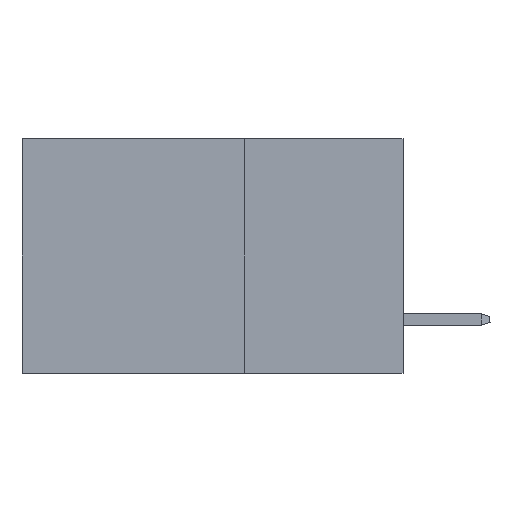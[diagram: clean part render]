
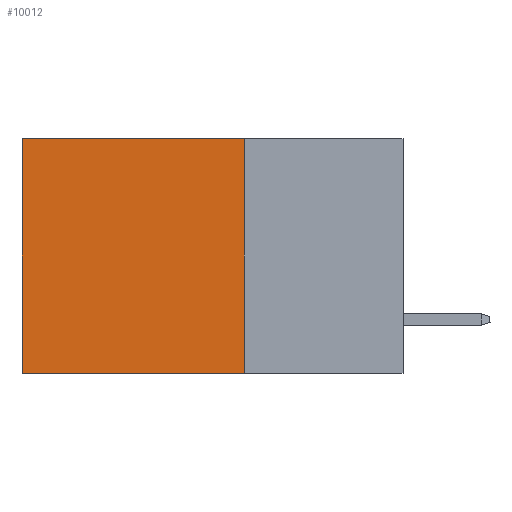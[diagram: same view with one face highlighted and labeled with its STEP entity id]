
A CAD part, left-side view. The second image highlights one B-rep face of the part: STEP entity #10012.
In plain terms, the highlighted planar face has unit normal (-1, 0, 0).
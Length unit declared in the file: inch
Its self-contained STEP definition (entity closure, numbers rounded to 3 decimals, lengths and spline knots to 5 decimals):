
#1174 = DIRECTION ( 'NONE',  ( 0., 1., 0. ) ) ;
#1626 = VERTEX_POINT ( 'NONE', #35680 ) ;
#2067 = LINE ( 'NONE', #16217, #13193 ) ;
#4987 = VECTOR ( 'NONE', #1174, 39.37008 ) ;
#7711 = CARTESIAN_POINT ( 'NONE',  ( 0.2875, 0.25, 0. ) ) ;
#7840 = EDGE_CURVE ( 'NONE', #28309, #1626, #2067, .T. ) ;
#8248 = CARTESIAN_POINT ( 'NONE',  ( 0.2875, 0.25, 0. ) ) ;
#9407 = DIRECTION ( 'NONE',  ( 0., 0., -1. ) ) ;
#9444 = CARTESIAN_POINT ( 'NONE',  ( 0.2875, 0.6, -0.37 ) ) ;
#10012 = ADVANCED_FACE ( 'NONE', ( #19059 ), #16410, .F. ) ;
#12593 = LINE ( 'NONE', #29632, #17656 ) ;
#12969 = DIRECTION ( 'NONE',  ( 0., 1., 0. ) ) ;
#13193 = VECTOR ( 'NONE', #36003, 39.37008 ) ;
#13343 = CARTESIAN_POINT ( 'NONE',  ( 0.2875, 0.25, 0. ) ) ;
#14659 = EDGE_CURVE ( 'NONE', #28309, #22781, #18462, .T. ) ;
#15613 = CARTESIAN_POINT ( 'NONE',  ( 0.2875, 0.6, 0. ) ) ;
#15822 = EDGE_CURVE ( 'NONE', #22781, #23527, #12593, .T. ) ;
#16217 = CARTESIAN_POINT ( 'NONE',  ( 0.2875, 0.25, 0. ) ) ;
#16410 = PLANE ( 'NONE',  #28434 ) ;
#17656 = VECTOR ( 'NONE', #9407, 39.37008 ) ;
#18462 = LINE ( 'NONE', #13343, #32437 ) ;
#19059 = FACE_OUTER_BOUND ( 'NONE', #37117, .T. ) ;
#19250 = DIRECTION ( 'NONE',  ( 0., 0., -1. ) ) ;
#22781 = VERTEX_POINT ( 'NONE', #15613 ) ;
#23527 = VERTEX_POINT ( 'NONE', #9444 ) ;
#27048 = CARTESIAN_POINT ( 'NONE',  ( 0.2875, 0.25, -0.37 ) ) ;
#28309 = VERTEX_POINT ( 'NONE', #8248 ) ;
#28434 = AXIS2_PLACEMENT_3D ( 'NONE', #7711, #36937, #19250 ) ;
#29013 = ORIENTED_EDGE ( 'NONE', *, *, #7840, .F. ) ;
#29632 = CARTESIAN_POINT ( 'NONE',  ( 0.2875, 0.6, 0. ) ) ;
#32437 = VECTOR ( 'NONE', #12969, 39.37008 ) ;
#32863 = LINE ( 'NONE', #27048, #4987 ) ;
#33533 = ORIENTED_EDGE ( 'NONE', *, *, #36767, .F. ) ;
#33641 = ORIENTED_EDGE ( 'NONE', *, *, #15822, .T. ) ;
#35680 = CARTESIAN_POINT ( 'NONE',  ( 0.2875, 0.25, -0.37 ) ) ;
#36003 = DIRECTION ( 'NONE',  ( 0., 0., -1. ) ) ;
#36396 = ORIENTED_EDGE ( 'NONE', *, *, #14659, .T. ) ;
#36767 = EDGE_CURVE ( 'NONE', #1626, #23527, #32863, .T. ) ;
#36937 = DIRECTION ( 'NONE',  ( 1., 0., 0. ) ) ;
#37117 = EDGE_LOOP ( 'NONE', ( #33641, #33533, #29013, #36396 ) ) ;
